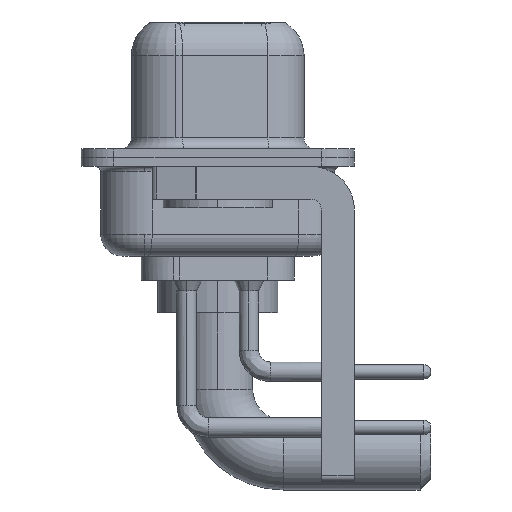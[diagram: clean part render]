
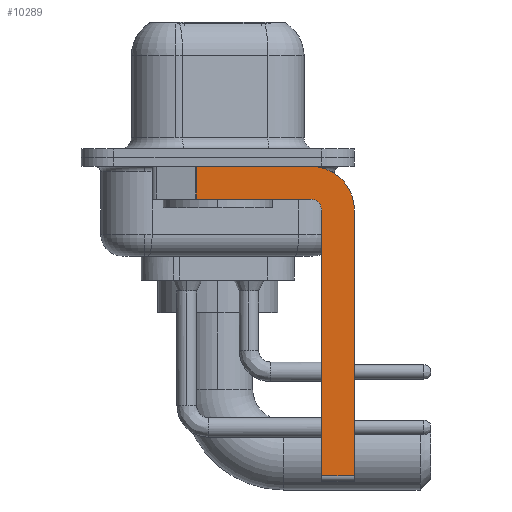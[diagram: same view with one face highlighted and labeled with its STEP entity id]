
A CAD part, left-side view. The second image highlights one B-rep face of the part: STEP entity #10289.
In plain terms, the highlighted planar face has unit normal (-1, 0, 0).
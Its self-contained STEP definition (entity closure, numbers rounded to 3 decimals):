
#809 = ORIENTED_EDGE ( 'NONE', *, *, #1041, .T. ) ;
#1041 = EDGE_CURVE ( 'NONE', #13651, #5401, #1565, .T. ) ;
#1255 = CARTESIAN_POINT ( 'NONE',  ( -2.9, -6.25, -2.4 ) ) ;
#1413 = DIRECTION ( 'NONE',  ( 0., 0., 1. ) ) ;
#1565 = LINE ( 'NONE', #8184, #6479 ) ;
#1670 = CIRCLE ( 'NONE', #5515, 2. ) ;
#2070 = VERTEX_POINT ( 'NONE', #11074 ) ;
#2153 = LINE ( 'NONE', #7398, #14038 ) ;
#2477 = ORIENTED_EDGE ( 'NONE', *, *, #5473, .F. ) ;
#2661 = DIRECTION ( 'NONE',  ( 0., -1., 0. ) ) ;
#3226 = EDGE_CURVE ( 'NONE', #13651, #7043, #10239, .T. ) ;
#3475 = DIRECTION ( 'NONE',  ( 0., 0., -1. ) ) ;
#3571 = ORIENTED_EDGE ( 'NONE', *, *, #6175, .F. ) ;
#3607 = CARTESIAN_POINT ( 'NONE',  ( -2.9, 0.978, -1.9 ) ) ;
#3817 = VECTOR ( 'NONE', #3871, 1000. ) ;
#3871 = DIRECTION ( 'NONE',  ( 0., -1., 0. ) ) ;
#4676 = CARTESIAN_POINT ( 'NONE',  ( -2.9, -4.25, -2.4 ) ) ;
#5060 = VERTEX_POINT ( 'NONE', #10656 ) ;
#5401 = VERTEX_POINT ( 'NONE', #3607 ) ;
#5473 = EDGE_CURVE ( 'NONE', #14513, #5401, #9088, .T. ) ;
#5515 = AXIS2_PLACEMENT_3D ( 'NONE', #4676, #8628, #3475 ) ;
#5712 = CARTESIAN_POINT ( 'NONE',  ( -2.9, 0.978, -0.4 ) ) ;
#6175 = EDGE_CURVE ( 'NONE', #16797, #14513, #10700, .T. ) ;
#6427 = EDGE_CURVE ( 'NONE', #7513, #2070, #7070, .T. ) ;
#6431 = CARTESIAN_POINT ( 'NONE',  ( -2.9, -4.25, -1.9 ) ) ;
#6479 = VECTOR ( 'NONE', #13444, 1000. ) ;
#6526 = DIRECTION ( 'NONE',  ( 1., 0., 0. ) ) ;
#6718 = DIRECTION ( 'NONE',  ( 0., 0., -1. ) ) ;
#6942 = EDGE_CURVE ( 'NONE', #5060, #16797, #2153, .T. ) ;
#7024 = AXIS2_PLACEMENT_3D ( 'NONE', #10563, #6526, #15512 ) ;
#7043 = VERTEX_POINT ( 'NONE', #15927 ) ;
#7070 = LINE ( 'NONE', #13526, #13186 ) ;
#7398 = CARTESIAN_POINT ( 'NONE',  ( -2.9, -4.75, -14.8 ) ) ;
#7513 = VERTEX_POINT ( 'NONE', #1255 ) ;
#7736 = FACE_OUTER_BOUND ( 'NONE', #9989, .T. ) ;
#8184 = CARTESIAN_POINT ( 'NONE',  ( -2.9, 0.978, -1.9 ) ) ;
#8274 = CARTESIAN_POINT ( 'NONE',  ( -2.9, -4.75, -2.4 ) ) ;
#8424 = VECTOR ( 'NONE', #2661, 1000. ) ;
#8556 = ORIENTED_EDGE ( 'NONE', *, *, #6427, .F. ) ;
#8628 = DIRECTION ( 'NONE',  ( 1., 0., 0. ) ) ;
#8669 = ORIENTED_EDGE ( 'NONE', *, *, #6942, .F. ) ;
#8888 = ORIENTED_EDGE ( 'NONE', *, *, #11960, .F. ) ;
#9088 = LINE ( 'NONE', #6431, #12051 ) ;
#9231 = DIRECTION ( 'NONE',  ( -1., 0., 0. ) ) ;
#9584 = CARTESIAN_POINT ( 'NONE',  ( -2.9, -4.25, -2.4 ) ) ;
#9989 = EDGE_LOOP ( 'NONE', ( #15778, #809, #2477, #3571, #8669, #14162, #8556, #8888 ) ) ;
#10239 = LINE ( 'NONE', #12907, #3817 ) ;
#10289 = ADVANCED_FACE ( 'NONE', ( #7736 ), #12991, .F. ) ;
#10563 = CARTESIAN_POINT ( 'NONE',  ( -2.9, -4.25, -2.4 ) ) ;
#10656 = CARTESIAN_POINT ( 'NONE',  ( -2.9, -4.75, -14.55 ) ) ;
#10700 = CIRCLE ( 'NONE', #14560, 0.5 ) ;
#11074 = CARTESIAN_POINT ( 'NONE',  ( -2.9, -6.25, -14.55 ) ) ;
#11362 = EDGE_CURVE ( 'NONE', #5060, #2070, #16990, .T. ) ;
#11678 = DIRECTION ( 'NONE',  ( 0., 1., 0. ) ) ;
#11960 = EDGE_CURVE ( 'NONE', #7043, #7513, #1670, .T. ) ;
#12051 = VECTOR ( 'NONE', #11678, 1000. ) ;
#12645 = DIRECTION ( 'NONE',  ( 0., 0., 1. ) ) ;
#12907 = CARTESIAN_POINT ( 'NONE',  ( -2.9, 3., -0.4 ) ) ;
#12991 = PLANE ( 'NONE',  #7024 ) ;
#13186 = VECTOR ( 'NONE', #6718, 1000. ) ;
#13444 = DIRECTION ( 'NONE',  ( 0., 0., -1. ) ) ;
#13526 = CARTESIAN_POINT ( 'NONE',  ( -2.9, -6.25, -2.4 ) ) ;
#13651 = VERTEX_POINT ( 'NONE', #5712 ) ;
#14038 = VECTOR ( 'NONE', #12645, 1000. ) ;
#14162 = ORIENTED_EDGE ( 'NONE', *, *, #11362, .T. ) ;
#14513 = VERTEX_POINT ( 'NONE', #14524 ) ;
#14524 = CARTESIAN_POINT ( 'NONE',  ( -2.9, -4.25, -1.9 ) ) ;
#14560 = AXIS2_PLACEMENT_3D ( 'NONE', #9584, #9231, #1413 ) ;
#14718 = CARTESIAN_POINT ( 'NONE',  ( -2.9, -4.25, -14.55 ) ) ;
#15512 = DIRECTION ( 'NONE',  ( 0., 0., -1. ) ) ;
#15778 = ORIENTED_EDGE ( 'NONE', *, *, #3226, .F. ) ;
#15927 = CARTESIAN_POINT ( 'NONE',  ( -2.9, -4.25, -0.4 ) ) ;
#16797 = VERTEX_POINT ( 'NONE', #8274 ) ;
#16990 = LINE ( 'NONE', #14718, #8424 ) ;
